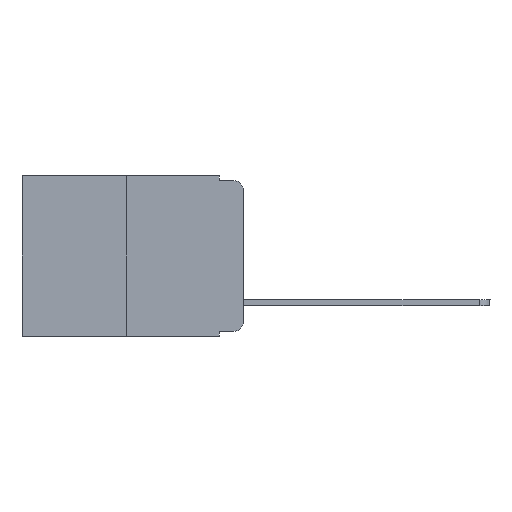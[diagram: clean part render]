
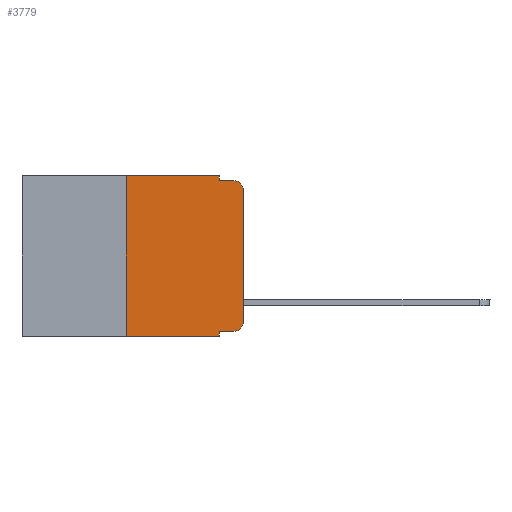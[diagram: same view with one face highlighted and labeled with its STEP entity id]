
A CAD part, left-side view. The second image highlights one B-rep face of the part: STEP entity #3779.
In plain terms, the highlighted planar face has unit normal (-1, 0, 0).
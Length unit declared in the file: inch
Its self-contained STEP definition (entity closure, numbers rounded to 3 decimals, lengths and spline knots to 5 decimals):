
#102 = CIRCLE ( 'NONE', #3318, 0.02 ) ;
#219 = LINE ( 'NONE', #4808, #1364 ) ;
#303 = DIRECTION ( 'NONE',  ( 0., -1., 0. ) ) ;
#408 = VECTOR ( 'NONE', #303, 39.37008 ) ;
#469 = EDGE_LOOP ( 'NONE', ( #993, #5522, #2597, #6785, #9079, #3777, #8557, #8627, #2399, #4353 ) ) ;
#476 = EDGE_CURVE ( 'NONE', #2222, #5245, #219, .T. ) ;
#477 = CARTESIAN_POINT ( 'NONE',  ( 0., 0.02, -0.313 ) ) ;
#548 = EDGE_CURVE ( 'NONE', #9015, #9639, #1071, .T. ) ;
#576 = VERTEX_POINT ( 'NONE', #3634 ) ;
#601 = DIRECTION ( 'NONE',  ( 0., 0., 1. ) ) ;
#784 = CARTESIAN_POINT ( 'NONE',  ( 0., 0.051, -0.01 ) ) ;
#834 = CARTESIAN_POINT ( 'NONE',  ( 0., 0.02, -0.03 ) ) ;
#878 = DIRECTION ( 'NONE',  ( 0., 0., -1. ) ) ;
#955 = EDGE_CURVE ( 'NONE', #7332, #9759, #1048, .T. ) ;
#993 = ORIENTED_EDGE ( 'NONE', *, *, #548, .T. ) ;
#1048 = LINE ( 'NONE', #4129, #408 ) ;
#1071 = LINE ( 'NONE', #1635, #3298 ) ;
#1135 = DIRECTION ( 'NONE',  ( 1., 0., 0. ) ) ;
#1364 = VECTOR ( 'NONE', #7844, 39.37008 ) ;
#1447 = VERTEX_POINT ( 'NONE', #8860 ) ;
#1500 = DIRECTION ( 'NONE',  ( -1., 0., 0. ) ) ;
#1560 = DIRECTION ( 'NONE',  ( 0., -1., 0. ) ) ;
#1578 = EDGE_CURVE ( 'NONE', #7332, #5245, #1639, .T. ) ;
#1635 = CARTESIAN_POINT ( 'NONE',  ( 0., 0., 0. ) ) ;
#1639 = LINE ( 'NONE', #2252, #2151 ) ;
#2010 = LINE ( 'NONE', #2161, #2466 ) ;
#2050 = DIRECTION ( 'NONE',  ( 0., 0., -1. ) ) ;
#2151 = VECTOR ( 'NONE', #878, 39.37008 ) ;
#2161 = CARTESIAN_POINT ( 'NONE',  ( 0., 0.051, 0. ) ) ;
#2222 = VERTEX_POINT ( 'NONE', #2815 ) ;
#2252 = CARTESIAN_POINT ( 'NONE',  ( 0., 0.051, 0. ) ) ;
#2267 = EDGE_CURVE ( 'NONE', #576, #7239, #2010, .T. ) ;
#2377 = EDGE_CURVE ( 'NONE', #1447, #576, #4725, .T. ) ;
#2399 = ORIENTED_EDGE ( 'NONE', *, *, #955, .T. ) ;
#2466 = VECTOR ( 'NONE', #4325, 39.37008 ) ;
#2597 = ORIENTED_EDGE ( 'NONE', *, *, #9694, .F. ) ;
#2599 = DIRECTION ( 'NONE',  ( 0., -1., 0. ) ) ;
#2815 = CARTESIAN_POINT ( 'NONE',  ( 0., 0.25, -0.343 ) ) ;
#2885 = CARTESIAN_POINT ( 'NONE',  ( 0., 0., -0.313 ) ) ;
#3298 = VECTOR ( 'NONE', #4710, 39.37008 ) ;
#3318 = AXIS2_PLACEMENT_3D ( 'NONE', #834, #1500, #7648 ) ;
#3356 = LINE ( 'NONE', #6428, #9757 ) ;
#3634 = CARTESIAN_POINT ( 'NONE',  ( 0., 0.051, 0. ) ) ;
#3777 = ORIENTED_EDGE ( 'NONE', *, *, #6552, .F. ) ;
#3779 = ADVANCED_FACE ( 'NONE', ( #5022 ), #8160, .F. ) ;
#4129 = CARTESIAN_POINT ( 'NONE',  ( 0., 0.051, -0.333 ) ) ;
#4325 = DIRECTION ( 'NONE',  ( 0., 0., -1. ) ) ;
#4353 = ORIENTED_EDGE ( 'NONE', *, *, #8471, .T. ) ;
#4710 = DIRECTION ( 'NONE',  ( 0., 0., 1. ) ) ;
#4725 = LINE ( 'NONE', #9175, #5670 ) ;
#4752 = VECTOR ( 'NONE', #601, 39.37008 ) ;
#4808 = CARTESIAN_POINT ( 'NONE',  ( 0., 0.473, -0.343 ) ) ;
#5004 = CARTESIAN_POINT ( 'NONE',  ( 0., 0.051, -0.333 ) ) ;
#5022 = FACE_OUTER_BOUND ( 'NONE', #469, .T. ) ;
#5183 = AXIS2_PLACEMENT_3D ( 'NONE', #8009, #1135, #8864 ) ;
#5245 = VERTEX_POINT ( 'NONE', #9120 ) ;
#5371 = VERTEX_POINT ( 'NONE', #6182 ) ;
#5522 = ORIENTED_EDGE ( 'NONE', *, *, #9518, .T. ) ;
#5541 = AXIS2_PLACEMENT_3D ( 'NONE', #477, #8295, #2050 ) ;
#5620 = CARTESIAN_POINT ( 'NONE',  ( 0., 0., -0.03 ) ) ;
#5670 = VECTOR ( 'NONE', #1560, 39.37008 ) ;
#6182 = CARTESIAN_POINT ( 'NONE',  ( 0., 0.02, -0.01 ) ) ;
#6428 = CARTESIAN_POINT ( 'NONE',  ( 0., 0.051, -0.01 ) ) ;
#6552 = EDGE_CURVE ( 'NONE', #2222, #1447, #8411, .T. ) ;
#6785 = ORIENTED_EDGE ( 'NONE', *, *, #2267, .F. ) ;
#7239 = VERTEX_POINT ( 'NONE', #784 ) ;
#7332 = VERTEX_POINT ( 'NONE', #5004 ) ;
#7648 = DIRECTION ( 'NONE',  ( 0., 0., -1. ) ) ;
#7833 = CIRCLE ( 'NONE', #5541, 0.02 ) ;
#7844 = DIRECTION ( 'NONE',  ( 0., -1., 0. ) ) ;
#8009 = CARTESIAN_POINT ( 'NONE',  ( 0., 0.473, 0. ) ) ;
#8160 = PLANE ( 'NONE',  #5183 ) ;
#8295 = DIRECTION ( 'NONE',  ( -1., 0., 0. ) ) ;
#8411 = LINE ( 'NONE', #9176, #4752 ) ;
#8471 = EDGE_CURVE ( 'NONE', #9759, #9015, #7833, .T. ) ;
#8557 = ORIENTED_EDGE ( 'NONE', *, *, #476, .T. ) ;
#8627 = ORIENTED_EDGE ( 'NONE', *, *, #1578, .F. ) ;
#8860 = CARTESIAN_POINT ( 'NONE',  ( 0., 0.25, 0. ) ) ;
#8864 = DIRECTION ( 'NONE',  ( 0., 0., -1. ) ) ;
#9004 = CARTESIAN_POINT ( 'NONE',  ( 0., 0.02, -0.333 ) ) ;
#9015 = VERTEX_POINT ( 'NONE', #2885 ) ;
#9079 = ORIENTED_EDGE ( 'NONE', *, *, #2377, .F. ) ;
#9120 = CARTESIAN_POINT ( 'NONE',  ( 0., 0.051, -0.343 ) ) ;
#9175 = CARTESIAN_POINT ( 'NONE',  ( 0., 0.473, 0. ) ) ;
#9176 = CARTESIAN_POINT ( 'NONE',  ( 0., 0.25, 0. ) ) ;
#9518 = EDGE_CURVE ( 'NONE', #9639, #5371, #102, .T. ) ;
#9639 = VERTEX_POINT ( 'NONE', #5620 ) ;
#9694 = EDGE_CURVE ( 'NONE', #7239, #5371, #3356, .T. ) ;
#9757 = VECTOR ( 'NONE', #2599, 39.37008 ) ;
#9759 = VERTEX_POINT ( 'NONE', #9004 ) ;
